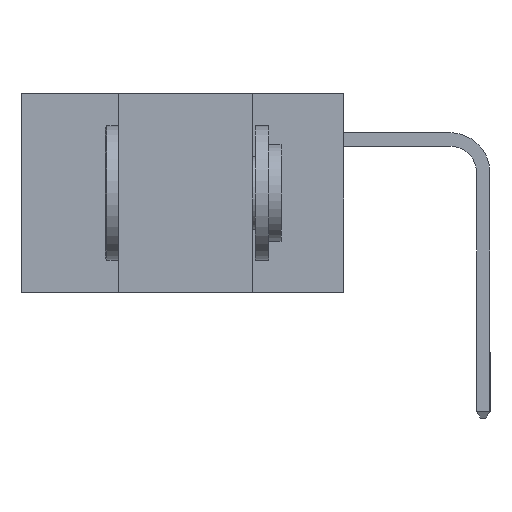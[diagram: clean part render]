
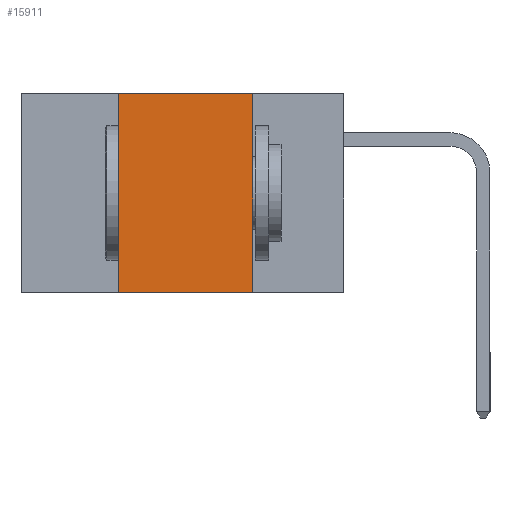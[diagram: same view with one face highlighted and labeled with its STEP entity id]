
A CAD part, left-side view. The second image highlights one B-rep face of the part: STEP entity #15911.
In plain terms, the highlighted planar face has unit normal (-1, 0, 0).
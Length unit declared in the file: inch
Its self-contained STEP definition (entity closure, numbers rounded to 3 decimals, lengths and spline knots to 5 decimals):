
#453 = VECTOR ( 'NONE', #16451, 39.37008 ) ;
#2218 = EDGE_CURVE ( 'NONE', #19092, #4361, #3679, .T. ) ;
#3627 = VECTOR ( 'NONE', #17655, 39.37008 ) ;
#3679 = LINE ( 'NONE', #5447, #453 ) ;
#4353 = VERTEX_POINT ( 'NONE', #17981 ) ;
#4361 = VERTEX_POINT ( 'NONE', #19975 ) ;
#4431 = PLANE ( 'NONE',  #21755 ) ;
#4513 = DIRECTION ( 'NONE',  ( 0., 0., -1. ) ) ;
#4875 = EDGE_CURVE ( 'NONE', #4353, #19092, #16613, .T. ) ;
#4931 = EDGE_CURVE ( 'NONE', #4361, #9186, #21595, .T. ) ;
#5447 = CARTESIAN_POINT ( 'NONE',  ( 0., 0.6, 0. ) ) ;
#5488 = ORIENTED_EDGE ( 'NONE', *, *, #2218, .F. ) ;
#5586 = FACE_OUTER_BOUND ( 'NONE', #21914, .T. ) ;
#5915 = CARTESIAN_POINT ( 'NONE',  ( 0., 0.17, 0. ) ) ;
#6798 = ORIENTED_EDGE ( 'NONE', *, *, #4875, .F. ) ;
#7659 = VECTOR ( 'NONE', #17319, 39.37008 ) ;
#7798 = CARTESIAN_POINT ( 'NONE',  ( 0., 0.42, 0. ) ) ;
#9186 = VERTEX_POINT ( 'NONE', #14666 ) ;
#9818 = CARTESIAN_POINT ( 'NONE',  ( 0., 0.42, 0. ) ) ;
#10291 = DIRECTION ( 'NONE',  ( 0., 0., -1. ) ) ;
#10788 = ORIENTED_EDGE ( 'NONE', *, *, #4931, .F. ) ;
#13528 = CARTESIAN_POINT ( 'NONE',  ( 0., 0.6, 0. ) ) ;
#13691 = DIRECTION ( 'NONE',  ( 1., 0., 0. ) ) ;
#14048 = VECTOR ( 'NONE', #10291, 39.37008 ) ;
#14129 = EDGE_CURVE ( 'NONE', #4353, #9186, #22805, .T. ) ;
#14666 = CARTESIAN_POINT ( 'NONE',  ( 0., 0.17, -0.37 ) ) ;
#15911 = ADVANCED_FACE ( 'NONE', ( #5586 ), #4431, .F. ) ;
#16451 = DIRECTION ( 'NONE',  ( 0., -1., 0. ) ) ;
#16613 = LINE ( 'NONE', #9818, #7659 ) ;
#17319 = DIRECTION ( 'NONE',  ( 0., 0., 1. ) ) ;
#17655 = DIRECTION ( 'NONE',  ( 0., -1., 0. ) ) ;
#17981 = CARTESIAN_POINT ( 'NONE',  ( 0., 0.42, -0.37 ) ) ;
#19092 = VERTEX_POINT ( 'NONE', #7798 ) ;
#19448 = CARTESIAN_POINT ( 'NONE',  ( 0., 0.6, -0.37 ) ) ;
#19975 = CARTESIAN_POINT ( 'NONE',  ( 0., 0.17, 0. ) ) ;
#21595 = LINE ( 'NONE', #5915, #14048 ) ;
#21657 = ORIENTED_EDGE ( 'NONE', *, *, #14129, .T. ) ;
#21755 = AXIS2_PLACEMENT_3D ( 'NONE', #13528, #13691, #4513 ) ;
#21914 = EDGE_LOOP ( 'NONE', ( #10788, #5488, #6798, #21657 ) ) ;
#22805 = LINE ( 'NONE', #19448, #3627 ) ;
